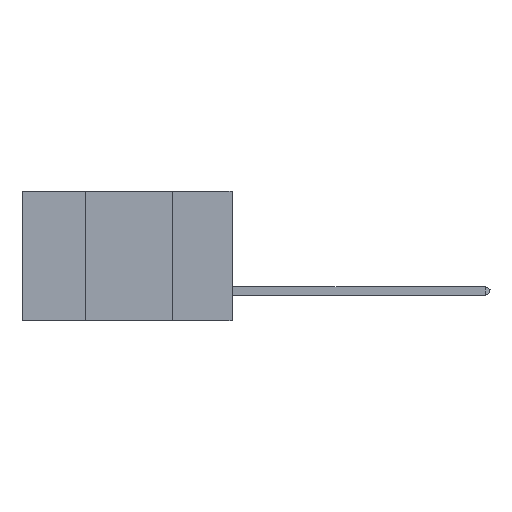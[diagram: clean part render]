
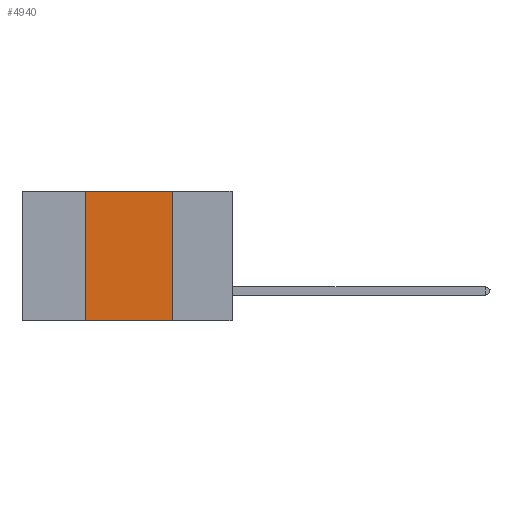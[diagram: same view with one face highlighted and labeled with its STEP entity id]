
A CAD part, left-side view. The second image highlights one B-rep face of the part: STEP entity #4940.
In plain terms, the highlighted planar face has unit normal (-1, 0, 0).
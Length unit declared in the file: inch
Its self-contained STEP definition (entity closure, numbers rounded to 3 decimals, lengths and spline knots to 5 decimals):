
#409 = VECTOR ( 'NONE', #3759, 39.37008 ) ;
#460 = CARTESIAN_POINT ( 'NONE',  ( 0., 0.17, 0. ) ) ;
#669 = LINE ( 'NONE', #460, #409 ) ;
#1502 = DIRECTION ( 'NONE',  ( 0., -1., 0. ) ) ;
#2359 = ORIENTED_EDGE ( 'NONE', *, *, #19410, .F. ) ;
#2727 = CARTESIAN_POINT ( 'NONE',  ( 0., 0.6, 0. ) ) ;
#3565 = ORIENTED_EDGE ( 'NONE', *, *, #18825, .T. ) ;
#3759 = DIRECTION ( 'NONE',  ( 0., 0., -1. ) ) ;
#3961 = DIRECTION ( 'NONE',  ( 1., 0., 0. ) ) ;
#4060 = CARTESIAN_POINT ( 'NONE',  ( 0., 0.17, 0. ) ) ;
#4184 = EDGE_CURVE ( 'NONE', #4539, #14102, #15659, .T. ) ;
#4539 = VERTEX_POINT ( 'NONE', #12448 ) ;
#4940 = ADVANCED_FACE ( 'NONE', ( #18152 ), #16654, .F. ) ;
#5605 = CARTESIAN_POINT ( 'NONE',  ( 0., 0.6, 0. ) ) ;
#5781 = CARTESIAN_POINT ( 'NONE',  ( 0., 0.42, -0.37 ) ) ;
#6394 = CARTESIAN_POINT ( 'NONE',  ( 0., 0.17, -0.37 ) ) ;
#8810 = EDGE_CURVE ( 'NONE', #14102, #10481, #669, .T. ) ;
#10481 = VERTEX_POINT ( 'NONE', #6394 ) ;
#11122 = LINE ( 'NONE', #19429, #11619 ) ;
#11466 = DIRECTION ( 'NONE',  ( 0., 0., 1. ) ) ;
#11583 = VECTOR ( 'NONE', #11466, 39.37008 ) ;
#11619 = VECTOR ( 'NONE', #1502, 39.37008 ) ;
#12168 = VECTOR ( 'NONE', #12692, 39.37008 ) ;
#12246 = ORIENTED_EDGE ( 'NONE', *, *, #4184, .F. ) ;
#12448 = CARTESIAN_POINT ( 'NONE',  ( 0., 0.42, 0. ) ) ;
#12692 = DIRECTION ( 'NONE',  ( 0., -1., 0. ) ) ;
#13694 = DIRECTION ( 'NONE',  ( 0., 0., -1. ) ) ;
#14102 = VERTEX_POINT ( 'NONE', #4060 ) ;
#14703 = ORIENTED_EDGE ( 'NONE', *, *, #8810, .F. ) ;
#15258 = VERTEX_POINT ( 'NONE', #5781 ) ;
#15659 = LINE ( 'NONE', #2727, #12168 ) ;
#16654 = PLANE ( 'NONE',  #17923 ) ;
#17788 = CARTESIAN_POINT ( 'NONE',  ( 0., 0.42, 0. ) ) ;
#17923 = AXIS2_PLACEMENT_3D ( 'NONE', #5605, #3961, #13694 ) ;
#18152 = FACE_OUTER_BOUND ( 'NONE', #18372, .T. ) ;
#18372 = EDGE_LOOP ( 'NONE', ( #14703, #12246, #2359, #3565 ) ) ;
#18825 = EDGE_CURVE ( 'NONE', #15258, #10481, #11122, .T. ) ;
#19410 = EDGE_CURVE ( 'NONE', #15258, #4539, #19667, .T. ) ;
#19429 = CARTESIAN_POINT ( 'NONE',  ( 0., 0.6, -0.37 ) ) ;
#19667 = LINE ( 'NONE', #17788, #11583 ) ;
